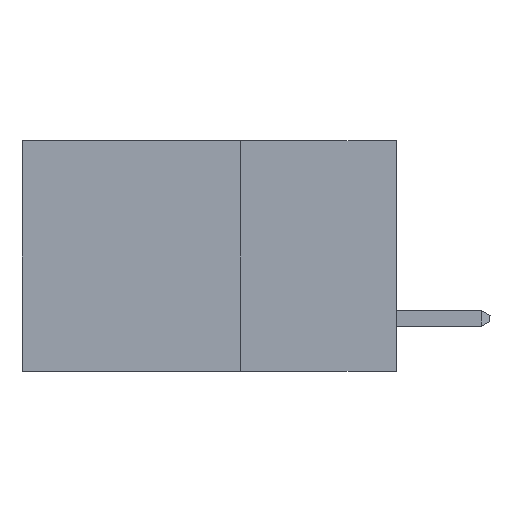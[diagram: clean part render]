
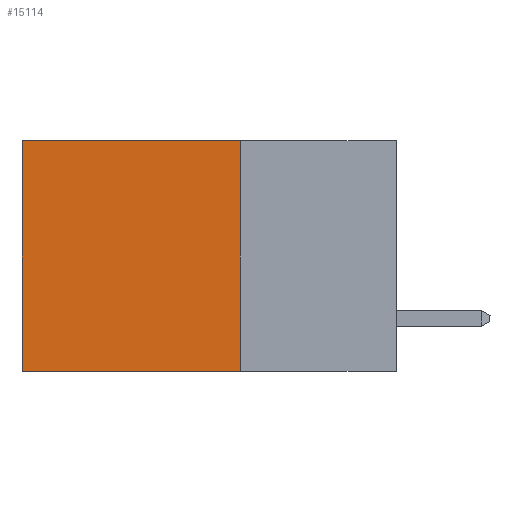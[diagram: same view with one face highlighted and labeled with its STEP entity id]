
A CAD part, left-side view. The second image highlights one B-rep face of the part: STEP entity #15114.
In plain terms, the highlighted planar face has unit normal (-1, 0, 0).
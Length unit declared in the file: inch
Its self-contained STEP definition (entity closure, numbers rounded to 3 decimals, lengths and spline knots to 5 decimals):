
#774 = CARTESIAN_POINT ( 'NONE',  ( 0.2615, 0.25, -0.37 ) ) ;
#1618 = EDGE_LOOP ( 'NONE', ( #11519, #13903, #11858, #12020 ) ) ;
#1788 = VERTEX_POINT ( 'NONE', #3262 ) ;
#2154 = EDGE_CURVE ( 'NONE', #10538, #6749, #18191, .T. ) ;
#3229 = DIRECTION ( 'NONE',  ( 1., 0., 0. ) ) ;
#3262 = CARTESIAN_POINT ( 'NONE',  ( 0.2615, 0.6, 0. ) ) ;
#3430 = FACE_OUTER_BOUND ( 'NONE', #1618, .T. ) ;
#4216 = VECTOR ( 'NONE', #7401, 39.37008 ) ;
#4620 = VECTOR ( 'NONE', #6152, 39.37008 ) ;
#4836 = EDGE_CURVE ( 'NONE', #1788, #8095, #8100, .T. ) ;
#5444 = VECTOR ( 'NONE', #11816, 39.37008 ) ;
#6152 = DIRECTION ( 'NONE',  ( 0., 0., -1. ) ) ;
#6749 = VERTEX_POINT ( 'NONE', #774 ) ;
#6918 = CARTESIAN_POINT ( 'NONE',  ( 0.2615, 0.6, -0.37 ) ) ;
#7401 = DIRECTION ( 'NONE',  ( 0., 1., 0. ) ) ;
#8095 = VERTEX_POINT ( 'NONE', #6918 ) ;
#8100 = LINE ( 'NONE', #15180, #13075 ) ;
#9374 = PLANE ( 'NONE',  #17940 ) ;
#9568 = DIRECTION ( 'NONE',  ( 0., 0., -1. ) ) ;
#9655 = EDGE_CURVE ( 'NONE', #10538, #1788, #19172, .T. ) ;
#10526 = LINE ( 'NONE', #16414, #4216 ) ;
#10538 = VERTEX_POINT ( 'NONE', #10771 ) ;
#10642 = CARTESIAN_POINT ( 'NONE',  ( 0.2615, 0.25, 0. ) ) ;
#10771 = CARTESIAN_POINT ( 'NONE',  ( 0.2615, 0.25, 0. ) ) ;
#11519 = ORIENTED_EDGE ( 'NONE', *, *, #4836, .T. ) ;
#11816 = DIRECTION ( 'NONE',  ( 0., 1., 0. ) ) ;
#11858 = ORIENTED_EDGE ( 'NONE', *, *, #2154, .F. ) ;
#12020 = ORIENTED_EDGE ( 'NONE', *, *, #9655, .T. ) ;
#12170 = CARTESIAN_POINT ( 'NONE',  ( 0.2615, 0.25, -0.37 ) ) ;
#13075 = VECTOR ( 'NONE', #13819, 39.37008 ) ;
#13723 = CARTESIAN_POINT ( 'NONE',  ( 0.2615, 0.25, -0.37 ) ) ;
#13819 = DIRECTION ( 'NONE',  ( 0., 0., -1. ) ) ;
#13903 = ORIENTED_EDGE ( 'NONE', *, *, #19028, .F. ) ;
#15114 = ADVANCED_FACE ( 'NONE', ( #3430 ), #9374, .F. ) ;
#15180 = CARTESIAN_POINT ( 'NONE',  ( 0.2615, 0.6, -0.37 ) ) ;
#16414 = CARTESIAN_POINT ( 'NONE',  ( 0.2615, 0.25, -0.37 ) ) ;
#17940 = AXIS2_PLACEMENT_3D ( 'NONE', #12170, #3229, #9568 ) ;
#18191 = LINE ( 'NONE', #13723, #4620 ) ;
#19028 = EDGE_CURVE ( 'NONE', #6749, #8095, #10526, .T. ) ;
#19172 = LINE ( 'NONE', #10642, #5444 ) ;
